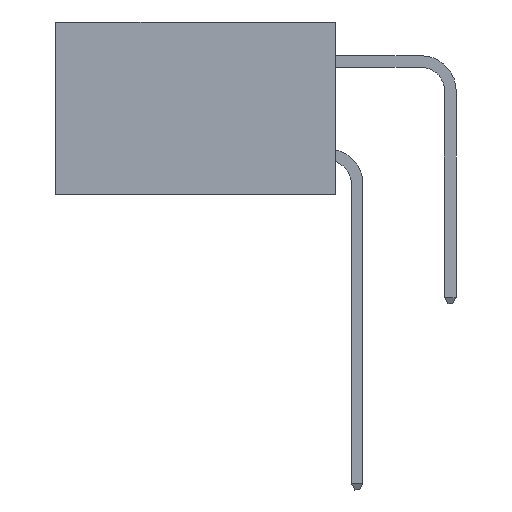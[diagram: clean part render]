
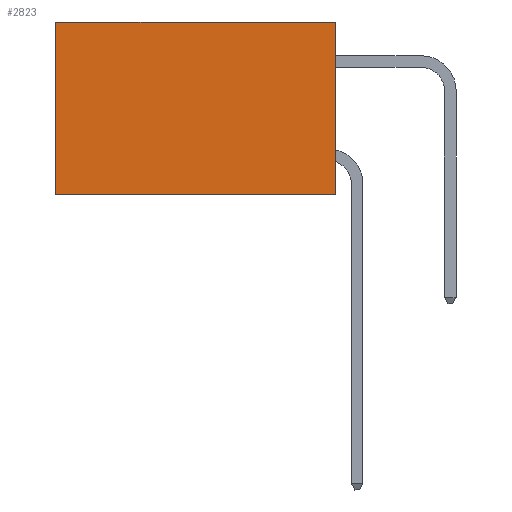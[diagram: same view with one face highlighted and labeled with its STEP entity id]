
A CAD part, left-side view. The second image highlights one B-rep face of the part: STEP entity #2823.
In plain terms, the highlighted planar face has unit normal (-1, 0, 0).
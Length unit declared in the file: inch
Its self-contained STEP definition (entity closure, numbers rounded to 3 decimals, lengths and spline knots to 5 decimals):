
#672 = EDGE_CURVE ( 'NONE', #28476, #12536, #15581, .T. ) ;
#2461 = ORIENTED_EDGE ( 'NONE', *, *, #17818, .T. ) ;
#2823 = ADVANCED_FACE ( 'NONE', ( #19200 ), #15353, .F. ) ;
#2866 = ORIENTED_EDGE ( 'NONE', *, *, #672, .T. ) ;
#3938 = CARTESIAN_POINT ( 'NONE',  ( 0.2875, 0., 0. ) ) ;
#4315 = DIRECTION ( 'NONE',  ( 1., 0., 0. ) ) ;
#4457 = CARTESIAN_POINT ( 'NONE',  ( 0.2875, 0.6, 0. ) ) ;
#4569 = VERTEX_POINT ( 'NONE', #5877 ) ;
#5877 = CARTESIAN_POINT ( 'NONE',  ( 0.2875, 0., -0.37 ) ) ;
#6089 = VECTOR ( 'NONE', #11111, 39.37008 ) ;
#6425 = LINE ( 'NONE', #22134, #6089 ) ;
#6507 = LINE ( 'NONE', #17074, #24141 ) ;
#6548 = DIRECTION ( 'NONE',  ( 0., 0., -1. ) ) ;
#8218 = DIRECTION ( 'NONE',  ( 0., 0., -1. ) ) ;
#8679 = CARTESIAN_POINT ( 'NONE',  ( 0.2875, 0., 0. ) ) ;
#9379 = VERTEX_POINT ( 'NONE', #3938 ) ;
#10474 = DIRECTION ( 'NONE',  ( 0., 1., 0. ) ) ;
#10701 = CARTESIAN_POINT ( 'NONE',  ( 0.2875, 0., 0. ) ) ;
#11111 = DIRECTION ( 'NONE',  ( 0., 1., 0. ) ) ;
#12536 = VERTEX_POINT ( 'NONE', #16857 ) ;
#14667 = LINE ( 'NONE', #8679, #26465 ) ;
#15353 = PLANE ( 'NONE',  #16387 ) ;
#15581 = LINE ( 'NONE', #25813, #19045 ) ;
#16387 = AXIS2_PLACEMENT_3D ( 'NONE', #10701, #4315, #6548 ) ;
#16857 = CARTESIAN_POINT ( 'NONE',  ( 0.2875, 0.6, -0.37 ) ) ;
#17074 = CARTESIAN_POINT ( 'NONE',  ( 0.2875, 0., -0.37 ) ) ;
#17818 = EDGE_CURVE ( 'NONE', #9379, #28476, #6425, .T. ) ;
#19045 = VECTOR ( 'NONE', #8218, 39.37008 ) ;
#19200 = FACE_OUTER_BOUND ( 'NONE', #21635, .T. ) ;
#21635 = EDGE_LOOP ( 'NONE', ( #2866, #21940, #22329, #2461 ) ) ;
#21940 = ORIENTED_EDGE ( 'NONE', *, *, #25055, .F. ) ;
#22134 = CARTESIAN_POINT ( 'NONE',  ( 0.2875, 0., 0. ) ) ;
#22329 = ORIENTED_EDGE ( 'NONE', *, *, #26989, .F. ) ;
#23933 = DIRECTION ( 'NONE',  ( 0., 0., -1. ) ) ;
#24141 = VECTOR ( 'NONE', #10474, 39.37008 ) ;
#25055 = EDGE_CURVE ( 'NONE', #4569, #12536, #6507, .T. ) ;
#25813 = CARTESIAN_POINT ( 'NONE',  ( 0.2875, 0.6, 0. ) ) ;
#26465 = VECTOR ( 'NONE', #23933, 39.37008 ) ;
#26989 = EDGE_CURVE ( 'NONE', #9379, #4569, #14667, .T. ) ;
#28476 = VERTEX_POINT ( 'NONE', #4457 ) ;
